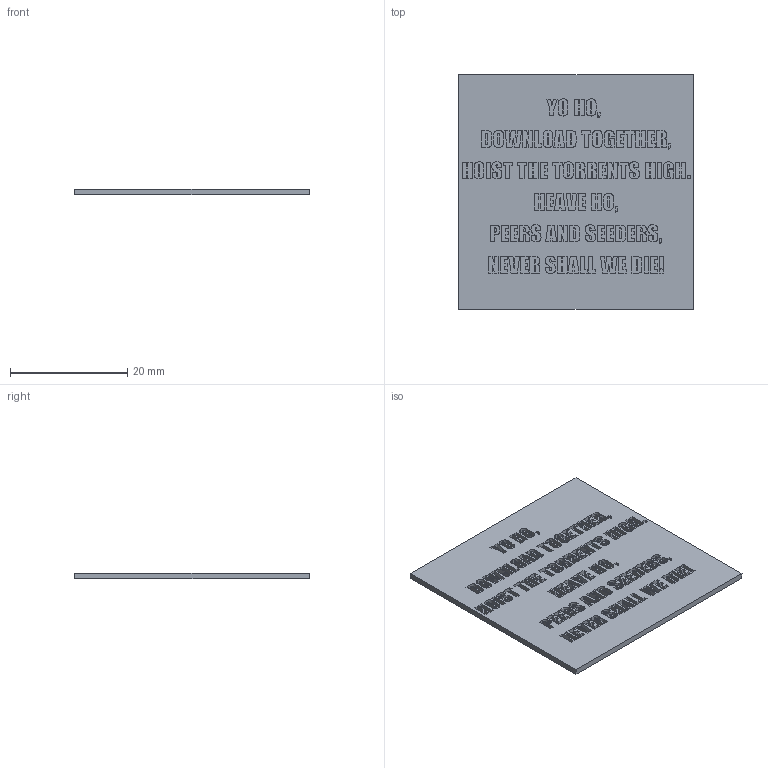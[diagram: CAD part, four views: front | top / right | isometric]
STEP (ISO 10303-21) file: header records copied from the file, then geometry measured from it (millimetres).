
FILE_DESCRIPTION (( 'STEP AP214' ), '1' );
FILE_NAME ('Hoist_The_Colours.STEP', '2013-09-01T23:25:51', ( 'Asher' ), ( '' ), 'SwSTEP 2.0', 'SolidWorks 2013', '' );
FILE_SCHEMA (( 'AUTOMOTIVE_DESIGN' ));
Length unit declared in the file: millimetre
Products named in the file (1): Hoist_The_Colours
Bounding box: 40 x 40 x 1 mm (x, y, z)
Volume: 1394.5 mm3; surface area: 4050.6 mm2
Topology: 1 solids, 1 shells, 1074 faces, 2892 edges, 1928 vertices
Faces by surface type: plane 811, bspline 263
Entity records: 48268 total; most frequent: CARTESIAN_POINT 23054, ORIENTED_EDGE 5784, DIRECTION 3990, EDGE_CURVE 2892, LINE 2366, VECTOR 2366, VERTEX_POINT 1928, EDGE_LOOP 1182
